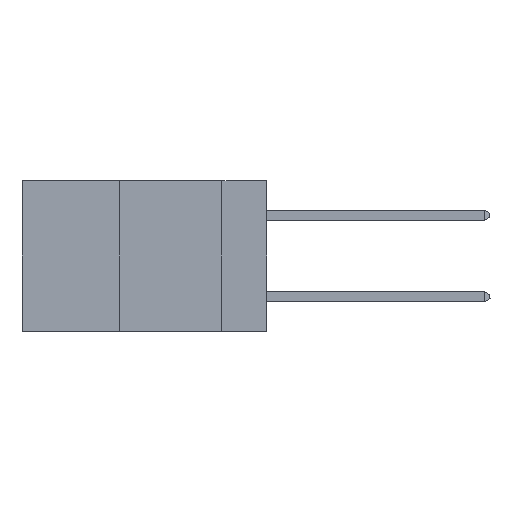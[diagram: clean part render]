
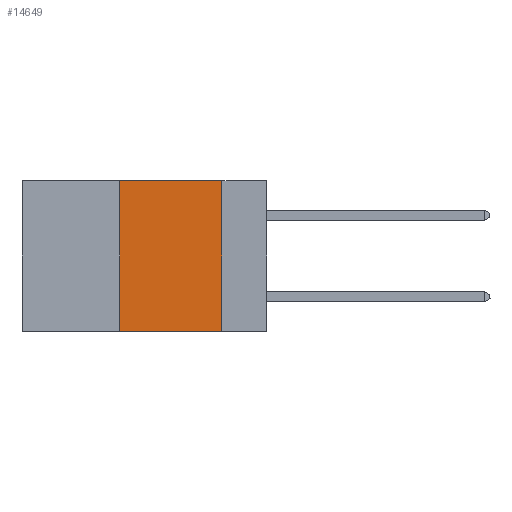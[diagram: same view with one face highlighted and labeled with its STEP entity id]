
A CAD part, left-side view. The second image highlights one B-rep face of the part: STEP entity #14649.
In plain terms, the highlighted planar face has unit normal (-1, 0, 0).
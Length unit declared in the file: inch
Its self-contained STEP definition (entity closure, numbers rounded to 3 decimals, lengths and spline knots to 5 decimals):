
#624 = LINE ( 'NONE', #6523, #8313 ) ;
#1001 = AXIS2_PLACEMENT_3D ( 'NONE', #23457, #26049, #15412 ) ;
#1833 = EDGE_CURVE ( 'NONE', #15134, #10465, #6397, .T. ) ;
#2827 = PLANE ( 'NONE',  #1001 ) ;
#3889 = VERTEX_POINT ( 'NONE', #11874 ) ;
#5883 = ORIENTED_EDGE ( 'NONE', *, *, #1833, .F. ) ;
#6145 = CARTESIAN_POINT ( 'NONE',  ( 0., 0.36, 0. ) ) ;
#6397 = LINE ( 'NONE', #6145, #23469 ) ;
#6523 = CARTESIAN_POINT ( 'NONE',  ( 0., 0.6, 0. ) ) ;
#7095 = EDGE_CURVE ( 'NONE', #23189, #3889, #21952, .T. ) ;
#7762 = ORIENTED_EDGE ( 'NONE', *, *, #13721, .T. ) ;
#8313 = VECTOR ( 'NONE', #16438, 39.37008 ) ;
#9407 = ORIENTED_EDGE ( 'NONE', *, *, #7095, .F. ) ;
#9536 = EDGE_CURVE ( 'NONE', #10465, #23189, #624, .T. ) ;
#10465 = VERTEX_POINT ( 'NONE', #25076 ) ;
#11874 = CARTESIAN_POINT ( 'NONE',  ( 0., 0.11, -0.37 ) ) ;
#12044 = FACE_OUTER_BOUND ( 'NONE', #13467, .T. ) ;
#13467 = EDGE_LOOP ( 'NONE', ( #9407, #22989, #5883, #7762 ) ) ;
#13721 = EDGE_CURVE ( 'NONE', #15134, #3889, #23631, .T. ) ;
#14649 = ADVANCED_FACE ( 'NONE', ( #12044 ), #2827, .F. ) ;
#15134 = VERTEX_POINT ( 'NONE', #18721 ) ;
#15412 = DIRECTION ( 'NONE',  ( 0., 0., -1. ) ) ;
#16381 = DIRECTION ( 'NONE',  ( 0., 0., -1. ) ) ;
#16438 = DIRECTION ( 'NONE',  ( 0., -1., 0. ) ) ;
#17772 = DIRECTION ( 'NONE',  ( 0., -1., 0. ) ) ;
#18721 = CARTESIAN_POINT ( 'NONE',  ( 0., 0.36, -0.37 ) ) ;
#20652 = DIRECTION ( 'NONE',  ( 0., 0., 1. ) ) ;
#21702 = VECTOR ( 'NONE', #17772, 39.37008 ) ;
#21952 = LINE ( 'NONE', #26251, #24187 ) ;
#22254 = CARTESIAN_POINT ( 'NONE',  ( 0., 0.6, -0.37 ) ) ;
#22989 = ORIENTED_EDGE ( 'NONE', *, *, #9536, .F. ) ;
#23189 = VERTEX_POINT ( 'NONE', #24952 ) ;
#23457 = CARTESIAN_POINT ( 'NONE',  ( 0., 0.6, 0. ) ) ;
#23469 = VECTOR ( 'NONE', #20652, 39.37008 ) ;
#23631 = LINE ( 'NONE', #22254, #21702 ) ;
#24187 = VECTOR ( 'NONE', #16381, 39.37008 ) ;
#24952 = CARTESIAN_POINT ( 'NONE',  ( 0., 0.11, 0. ) ) ;
#25076 = CARTESIAN_POINT ( 'NONE',  ( 0., 0.36, 0. ) ) ;
#26049 = DIRECTION ( 'NONE',  ( 1., 0., 0. ) ) ;
#26251 = CARTESIAN_POINT ( 'NONE',  ( 0., 0.11, 0. ) ) ;
